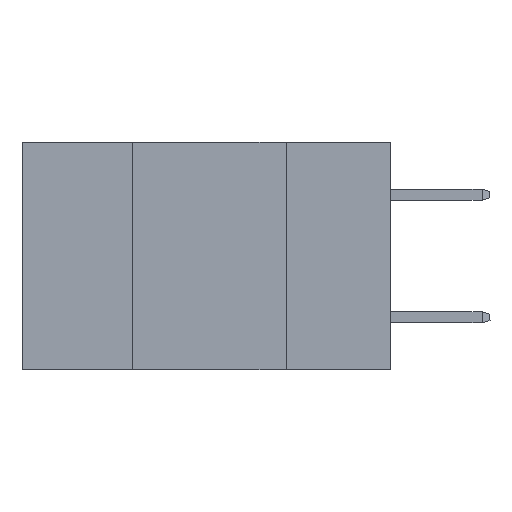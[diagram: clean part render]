
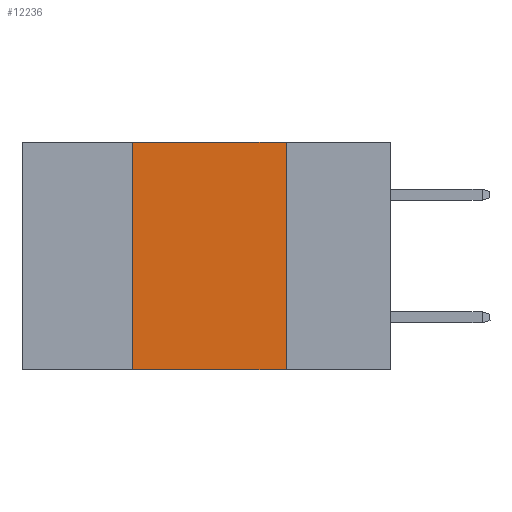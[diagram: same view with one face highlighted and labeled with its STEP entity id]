
A CAD part, left-side view. The second image highlights one B-rep face of the part: STEP entity #12236.
In plain terms, the highlighted planar face has unit normal (-1, 0, 0).
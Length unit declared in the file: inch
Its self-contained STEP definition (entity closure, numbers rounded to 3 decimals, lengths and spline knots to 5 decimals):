
#59 = DIRECTION ( 'NONE',  ( 0., 0., -1. ) ) ;
#1463 = EDGE_LOOP ( 'NONE', ( #5551, #9619, #14084, #18534 ) ) ;
#2038 = LINE ( 'NONE', #17767, #5587 ) ;
#2042 = LINE ( 'NONE', #19105, #10133 ) ;
#2319 = AXIS2_PLACEMENT_3D ( 'NONE', #6863, #16061, #6989 ) ;
#2767 = LINE ( 'NONE', #4912, #6294 ) ;
#3343 = VERTEX_POINT ( 'NONE', #15242 ) ;
#4912 = CARTESIAN_POINT ( 'NONE',  ( 0., 0.6, 0. ) ) ;
#4971 = FACE_OUTER_BOUND ( 'NONE', #1463, .T. ) ;
#5005 = VERTEX_POINT ( 'NONE', #18925 ) ;
#5272 = CARTESIAN_POINT ( 'NONE',  ( 0., 0.17, 0. ) ) ;
#5512 = DIRECTION ( 'NONE',  ( 0., -1., 0. ) ) ;
#5551 = ORIENTED_EDGE ( 'NONE', *, *, #16177, .F. ) ;
#5587 = VECTOR ( 'NONE', #10416, 39.37008 ) ;
#6294 = VECTOR ( 'NONE', #9529, 39.37008 ) ;
#6808 = VERTEX_POINT ( 'NONE', #5272 ) ;
#6840 = VECTOR ( 'NONE', #59, 39.37008 ) ;
#6863 = CARTESIAN_POINT ( 'NONE',  ( 0., 0.6, 0. ) ) ;
#6989 = DIRECTION ( 'NONE',  ( 0., 0., -1. ) ) ;
#9075 = EDGE_CURVE ( 'NONE', #10969, #5005, #2038, .T. ) ;
#9529 = DIRECTION ( 'NONE',  ( 0., -1., 0. ) ) ;
#9619 = ORIENTED_EDGE ( 'NONE', *, *, #17607, .F. ) ;
#10133 = VECTOR ( 'NONE', #5512, 39.37008 ) ;
#10416 = DIRECTION ( 'NONE',  ( 0., 0., 1. ) ) ;
#10969 = VERTEX_POINT ( 'NONE', #16572 ) ;
#12236 = ADVANCED_FACE ( 'NONE', ( #4971 ), #13055, .F. ) ;
#13055 = PLANE ( 'NONE',  #2319 ) ;
#14084 = ORIENTED_EDGE ( 'NONE', *, *, #9075, .F. ) ;
#14896 = LINE ( 'NONE', #18142, #6840 ) ;
#15242 = CARTESIAN_POINT ( 'NONE',  ( 0., 0.17, -0.37 ) ) ;
#16061 = DIRECTION ( 'NONE',  ( 1., 0., 0. ) ) ;
#16177 = EDGE_CURVE ( 'NONE', #6808, #3343, #14896, .T. ) ;
#16572 = CARTESIAN_POINT ( 'NONE',  ( 0., 0.42, -0.37 ) ) ;
#17607 = EDGE_CURVE ( 'NONE', #5005, #6808, #2767, .T. ) ;
#17767 = CARTESIAN_POINT ( 'NONE',  ( 0., 0.42, 0. ) ) ;
#17865 = EDGE_CURVE ( 'NONE', #10969, #3343, #2042, .T. ) ;
#18142 = CARTESIAN_POINT ( 'NONE',  ( 0., 0.17, 0. ) ) ;
#18534 = ORIENTED_EDGE ( 'NONE', *, *, #17865, .T. ) ;
#18925 = CARTESIAN_POINT ( 'NONE',  ( 0., 0.42, 0. ) ) ;
#19105 = CARTESIAN_POINT ( 'NONE',  ( 0., 0.6, -0.37 ) ) ;
